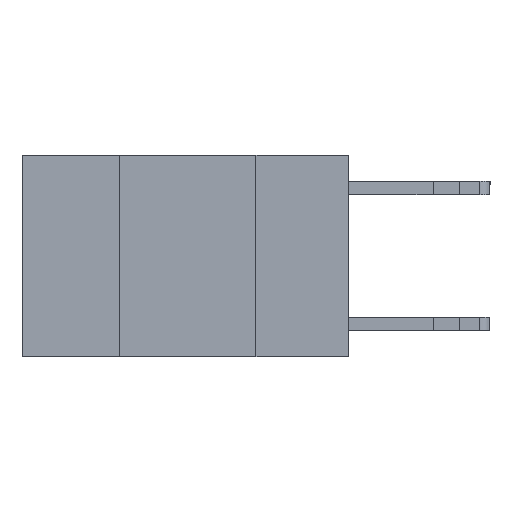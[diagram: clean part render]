
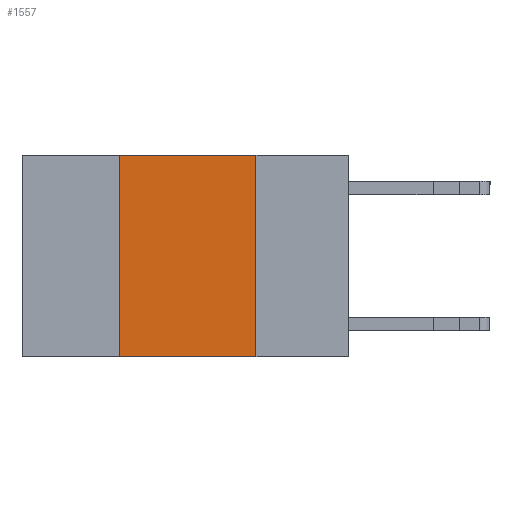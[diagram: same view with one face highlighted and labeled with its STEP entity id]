
A CAD part, left-side view. The second image highlights one B-rep face of the part: STEP entity #1557.
In plain terms, the highlighted planar face has unit normal (-1, 0, 0).
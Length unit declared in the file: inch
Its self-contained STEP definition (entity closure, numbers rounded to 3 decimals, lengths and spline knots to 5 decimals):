
#214 = VECTOR ( 'NONE', #4465, 39.37008 ) ;
#911 = CARTESIAN_POINT ( 'NONE',  ( 0., 0.42, 0. ) ) ;
#1129 = FACE_OUTER_BOUND ( 'NONE', #3059, .T. ) ;
#1210 = PLANE ( 'NONE',  #3258 ) ;
#1557 = ADVANCED_FACE ( 'NONE', ( #1129 ), #1210, .F. ) ;
#1717 = EDGE_CURVE ( 'NONE', #2865, #6958, #2975, .T. ) ;
#2245 = DIRECTION ( 'NONE',  ( 0., -1., 0. ) ) ;
#2643 = ORIENTED_EDGE ( 'NONE', *, *, #16504, .F. ) ;
#2865 = VERTEX_POINT ( 'NONE', #8798 ) ;
#2975 = LINE ( 'NONE', #13128, #15339 ) ;
#3059 = EDGE_LOOP ( 'NONE', ( #14242, #2643, #14954, #3167 ) ) ;
#3167 = ORIENTED_EDGE ( 'NONE', *, *, #6418, .T. ) ;
#3208 = DIRECTION ( 'NONE',  ( 0., -1., 0. ) ) ;
#3258 = AXIS2_PLACEMENT_3D ( 'NONE', #10442, #11790, #5105 ) ;
#4465 = DIRECTION ( 'NONE',  ( 0., 0., 1. ) ) ;
#5105 = DIRECTION ( 'NONE',  ( 0., 0., -1. ) ) ;
#5809 = LINE ( 'NONE', #9593, #12837 ) ;
#6116 = CARTESIAN_POINT ( 'NONE',  ( 0., 0.17, -0.37 ) ) ;
#6155 = VERTEX_POINT ( 'NONE', #11525 ) ;
#6418 = EDGE_CURVE ( 'NONE', #6155, #6958, #5809, .T. ) ;
#6913 = EDGE_CURVE ( 'NONE', #6155, #14096, #11166, .T. ) ;
#6958 = VERTEX_POINT ( 'NONE', #6116 ) ;
#7377 = LINE ( 'NONE', #9807, #8588 ) ;
#8588 = VECTOR ( 'NONE', #2245, 39.37008 ) ;
#8798 = CARTESIAN_POINT ( 'NONE',  ( 0., 0.17, 0. ) ) ;
#9593 = CARTESIAN_POINT ( 'NONE',  ( 0., 0.6, -0.37 ) ) ;
#9807 = CARTESIAN_POINT ( 'NONE',  ( 0., 0.6, 0. ) ) ;
#10442 = CARTESIAN_POINT ( 'NONE',  ( 0., 0.6, 0. ) ) ;
#11166 = LINE ( 'NONE', #12183, #214 ) ;
#11525 = CARTESIAN_POINT ( 'NONE',  ( 0., 0.42, -0.37 ) ) ;
#11790 = DIRECTION ( 'NONE',  ( 1., 0., 0. ) ) ;
#12183 = CARTESIAN_POINT ( 'NONE',  ( 0., 0.42, 0. ) ) ;
#12837 = VECTOR ( 'NONE', #3208, 39.37008 ) ;
#13128 = CARTESIAN_POINT ( 'NONE',  ( 0., 0.17, 0. ) ) ;
#13219 = DIRECTION ( 'NONE',  ( 0., 0., -1. ) ) ;
#14096 = VERTEX_POINT ( 'NONE', #911 ) ;
#14242 = ORIENTED_EDGE ( 'NONE', *, *, #1717, .F. ) ;
#14954 = ORIENTED_EDGE ( 'NONE', *, *, #6913, .F. ) ;
#15339 = VECTOR ( 'NONE', #13219, 39.37008 ) ;
#16504 = EDGE_CURVE ( 'NONE', #14096, #2865, #7377, .T. ) ;
